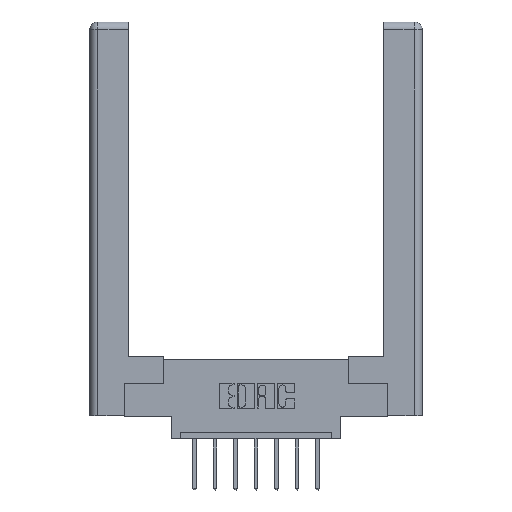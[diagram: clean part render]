
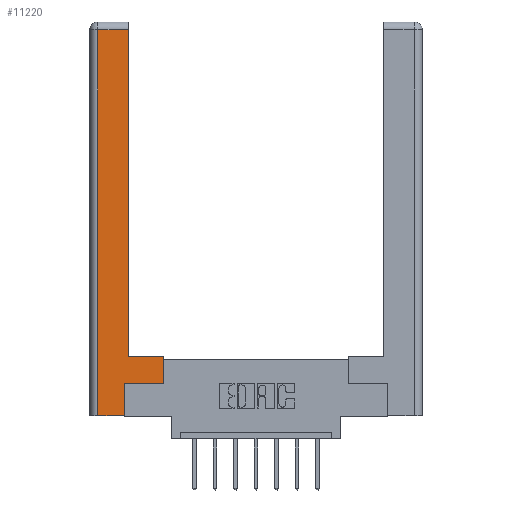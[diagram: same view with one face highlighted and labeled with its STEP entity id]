
A CAD part, top view. The second image highlights one B-rep face of the part: STEP entity #11220.
In plain terms, the highlighted planar face has unit normal (0, 0, 1).
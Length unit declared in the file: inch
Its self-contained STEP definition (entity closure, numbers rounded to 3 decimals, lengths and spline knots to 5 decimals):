
#43 = AXIS2_PLACEMENT_3D ( 'NONE', #1727, #11436, #5654 ) ;
#123 = VERTEX_POINT ( 'NONE', #2571 ) ;
#192 = VERTEX_POINT ( 'NONE', #5821 ) ;
#209 = DIRECTION ( 'NONE',  ( 1., 0., 0. ) ) ;
#407 = CARTESIAN_POINT ( 'NONE',  ( 0.0615, 0., 0. ) ) ;
#624 = CARTESIAN_POINT ( 'NONE',  ( 0.0615, 2.94, 0. ) ) ;
#700 = LINE ( 'NONE', #6137, #8301 ) ;
#1392 = EDGE_CURVE ( 'NONE', #6593, #123, #700, .T. ) ;
#1662 = VERTEX_POINT ( 'NONE', #624 ) ;
#1727 = CARTESIAN_POINT ( 'NONE',  ( 0., 0., 0. ) ) ;
#1859 = LINE ( 'NONE', #407, #2468 ) ;
#2033 = DIRECTION ( 'NONE',  ( -1., 0., 0. ) ) ;
#2083 = DIRECTION ( 'NONE',  ( 0., 1., 0. ) ) ;
#2193 = ORIENTED_EDGE ( 'NONE', *, *, #10474, .T. ) ;
#2317 = EDGE_CURVE ( 'NONE', #4787, #4469, #6918, .T. ) ;
#2358 = VECTOR ( 'NONE', #2033, 39.37008 ) ;
#2468 = VECTOR ( 'NONE', #8012, 39.37008 ) ;
#2571 = CARTESIAN_POINT ( 'NONE',  ( 0.295, 2.94, 0. ) ) ;
#2832 = VECTOR ( 'NONE', #2083, 39.37008 ) ;
#2926 = ORIENTED_EDGE ( 'NONE', *, *, #12364, .T. ) ;
#2966 = DIRECTION ( 'NONE',  ( 0., 1., 0. ) ) ;
#3012 = CARTESIAN_POINT ( 'NONE',  ( 0.565, 0.245, 0. ) ) ;
#3454 = LINE ( 'NONE', #3543, #9507 ) ;
#3459 = EDGE_CURVE ( 'NONE', #1662, #7440, #1859, .T. ) ;
#3516 = VERTEX_POINT ( 'NONE', #10906 ) ;
#3543 = CARTESIAN_POINT ( 'NONE',  ( 0.565, 0.245, 0. ) ) ;
#3675 = CARTESIAN_POINT ( 'NONE',  ( 0.0615, 0., 0. ) ) ;
#3750 = ORIENTED_EDGE ( 'NONE', *, *, #3459, .T. ) ;
#3771 = CARTESIAN_POINT ( 'NONE',  ( 0.295, 0.45, 0. ) ) ;
#4469 = VERTEX_POINT ( 'NONE', #5177 ) ;
#4733 = DIRECTION ( 'NONE',  ( -1., 0., 0. ) ) ;
#4787 = VERTEX_POINT ( 'NONE', #3012 ) ;
#4839 = CARTESIAN_POINT ( 'NONE',  ( 0.265, 0., 0. ) ) ;
#5136 = ORIENTED_EDGE ( 'NONE', *, *, #11278, .T. ) ;
#5177 = CARTESIAN_POINT ( 'NONE',  ( 0.565, 0.45, 0. ) ) ;
#5348 = ORIENTED_EDGE ( 'NONE', *, *, #11697, .T. ) ;
#5453 = LINE ( 'NONE', #3771, #11498 ) ;
#5654 = DIRECTION ( 'NONE',  ( -1., 0., 0. ) ) ;
#5805 = DIRECTION ( 'NONE',  ( 1., 0., 0. ) ) ;
#5821 = CARTESIAN_POINT ( 'NONE',  ( 0.265, 0.245, 0. ) ) ;
#5830 = CARTESIAN_POINT ( 'NONE',  ( 0.0615, 2.94, 0. ) ) ;
#5927 = CARTESIAN_POINT ( 'NONE',  ( 0.265, 0.245, 0. ) ) ;
#6049 = CARTESIAN_POINT ( 'NONE',  ( 0.565, 0.45, 0. ) ) ;
#6053 = FACE_OUTER_BOUND ( 'NONE', #6396, .T. ) ;
#6137 = CARTESIAN_POINT ( 'NONE',  ( 0.295, 3., 0. ) ) ;
#6341 = ORIENTED_EDGE ( 'NONE', *, *, #9551, .T. ) ;
#6386 = CARTESIAN_POINT ( 'NONE',  ( 0.295, 0.45, 0. ) ) ;
#6396 = EDGE_LOOP ( 'NONE', ( #11695, #5348, #3750, #2193, #5136, #6341, #10600, #2926 ) ) ;
#6593 = VERTEX_POINT ( 'NONE', #6386 ) ;
#6918 = LINE ( 'NONE', #6049, #10195 ) ;
#7440 = VERTEX_POINT ( 'NONE', #3675 ) ;
#7558 = PLANE ( 'NONE',  #43 ) ;
#8012 = DIRECTION ( 'NONE',  ( 0., -1., 0. ) ) ;
#8301 = VECTOR ( 'NONE', #9930, 39.37008 ) ;
#9332 = LINE ( 'NONE', #5927, #2832 ) ;
#9492 = LINE ( 'NONE', #4839, #10097 ) ;
#9507 = VECTOR ( 'NONE', #209, 39.37008 ) ;
#9551 = EDGE_CURVE ( 'NONE', #192, #4787, #3454, .T. ) ;
#9930 = DIRECTION ( 'NONE',  ( 0., 1., 0. ) ) ;
#10052 = LINE ( 'NONE', #5830, #2358 ) ;
#10097 = VECTOR ( 'NONE', #5805, 39.37008 ) ;
#10195 = VECTOR ( 'NONE', #2966, 39.37008 ) ;
#10474 = EDGE_CURVE ( 'NONE', #7440, #3516, #9492, .T. ) ;
#10600 = ORIENTED_EDGE ( 'NONE', *, *, #2317, .T. ) ;
#10906 = CARTESIAN_POINT ( 'NONE',  ( 0.265, 0., 0. ) ) ;
#11220 = ADVANCED_FACE ( 'NONE', ( #6053 ), #7558, .F. ) ;
#11278 = EDGE_CURVE ( 'NONE', #3516, #192, #9332, .T. ) ;
#11436 = DIRECTION ( 'NONE',  ( 0., 0., -1. ) ) ;
#11498 = VECTOR ( 'NONE', #4733, 39.37008 ) ;
#11695 = ORIENTED_EDGE ( 'NONE', *, *, #1392, .T. ) ;
#11697 = EDGE_CURVE ( 'NONE', #123, #1662, #10052, .T. ) ;
#12364 = EDGE_CURVE ( 'NONE', #4469, #6593, #5453, .T. ) ;
